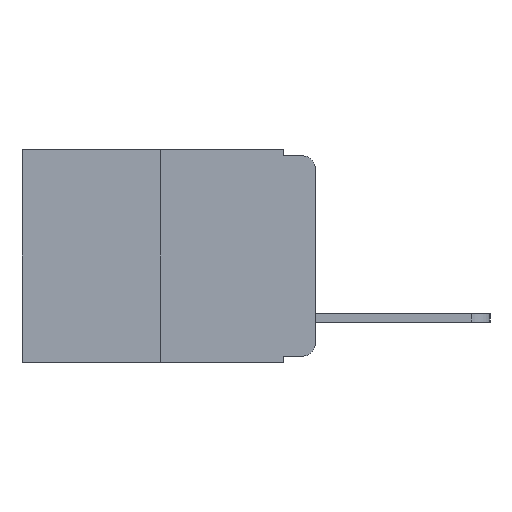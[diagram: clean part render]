
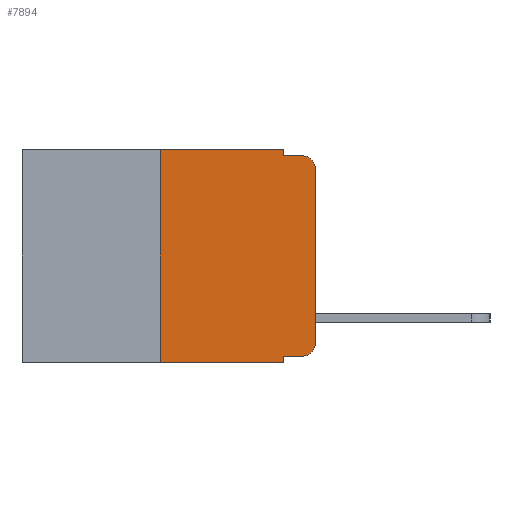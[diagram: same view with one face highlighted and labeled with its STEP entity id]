
A CAD part, left-side view. The second image highlights one B-rep face of the part: STEP entity #7894.
In plain terms, the highlighted planar face has unit normal (-1, 0, 0).
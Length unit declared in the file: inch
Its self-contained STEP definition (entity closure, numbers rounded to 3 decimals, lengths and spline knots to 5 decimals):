
#163 = AXIS2_PLACEMENT_3D ( 'NONE', #10218, #760, #6037 ) ;
#239 = EDGE_CURVE ( 'NONE', #9071, #713, #4498, .T. ) ;
#278 = VERTEX_POINT ( 'NONE', #9108 ) ;
#324 = VECTOR ( 'NONE', #2388, 39.37008 ) ;
#398 = DIRECTION ( 'NONE',  ( 0., 0., -1. ) ) ;
#529 = CARTESIAN_POINT ( 'NONE',  ( 0., 0.25, -0.343 ) ) ;
#713 = VERTEX_POINT ( 'NONE', #7970 ) ;
#725 = VERTEX_POINT ( 'NONE', #7679 ) ;
#760 = DIRECTION ( 'NONE',  ( 1., 0., 0. ) ) ;
#961 = EDGE_CURVE ( 'NONE', #4079, #9071, #7833, .T. ) ;
#1276 = FACE_OUTER_BOUND ( 'NONE', #2733, .T. ) ;
#1475 = LINE ( 'NONE', #11955, #6306 ) ;
#1564 = VERTEX_POINT ( 'NONE', #8216 ) ;
#1623 = PLANE ( 'NONE',  #163 ) ;
#2388 = DIRECTION ( 'NONE',  ( 0., 0., 1. ) ) ;
#2514 = LINE ( 'NONE', #10098, #7355 ) ;
#2542 = CARTESIAN_POINT ( 'NONE',  ( 0., 0., 0. ) ) ;
#2733 = EDGE_LOOP ( 'NONE', ( #9099, #9053, #7540, #7674, #8092, #8365, #9820, #9903, #7124, #10773 ) ) ;
#3201 = CARTESIAN_POINT ( 'NONE',  ( 0., 0.02, -0.333 ) ) ;
#3398 = VECTOR ( 'NONE', #6709, 39.37008 ) ;
#3698 = CARTESIAN_POINT ( 'NONE',  ( 0., 0.051, -0.01 ) ) ;
#4079 = VERTEX_POINT ( 'NONE', #12524 ) ;
#4468 = DIRECTION ( 'NONE',  ( 0., -1., 0. ) ) ;
#4474 = VERTEX_POINT ( 'NONE', #10710 ) ;
#4498 = CIRCLE ( 'NONE', #9310, 0.02 ) ;
#5006 = CARTESIAN_POINT ( 'NONE',  ( 0., 0.473, -0.343 ) ) ;
#5178 = VECTOR ( 'NONE', #5620, 39.37008 ) ;
#5368 = EDGE_CURVE ( 'NONE', #8167, #4474, #9248, .T. ) ;
#5620 = DIRECTION ( 'NONE',  ( 0., -1., 0. ) ) ;
#5674 = CARTESIAN_POINT ( 'NONE',  ( 0., 0.473, 0. ) ) ;
#5928 = CARTESIAN_POINT ( 'NONE',  ( 0., 0.051, 0. ) ) ;
#5963 = DIRECTION ( 'NONE',  ( 0., 0., -1. ) ) ;
#6037 = DIRECTION ( 'NONE',  ( 0., 0., -1. ) ) ;
#6229 = DIRECTION ( 'NONE',  ( 0., -1., 0. ) ) ;
#6306 = VECTOR ( 'NONE', #6229, 39.37008 ) ;
#6442 = EDGE_CURVE ( 'NONE', #7568, #4079, #12196, .T. ) ;
#6520 = CARTESIAN_POINT ( 'NONE',  ( 0., 0.02, -0.03 ) ) ;
#6709 = DIRECTION ( 'NONE',  ( 0., -1., 0. ) ) ;
#7108 = EDGE_CURVE ( 'NONE', #8213, #7568, #1475, .T. ) ;
#7124 = ORIENTED_EDGE ( 'NONE', *, *, #7108, .T. ) ;
#7355 = VECTOR ( 'NONE', #398, 39.37008 ) ;
#7428 = DIRECTION ( 'NONE',  ( 0., 0., -1. ) ) ;
#7532 = CARTESIAN_POINT ( 'NONE',  ( 0., 0.02, -0.313 ) ) ;
#7540 = ORIENTED_EDGE ( 'NONE', *, *, #11811, .F. ) ;
#7568 = VERTEX_POINT ( 'NONE', #3201 ) ;
#7674 = ORIENTED_EDGE ( 'NONE', *, *, #10619, .F. ) ;
#7679 = CARTESIAN_POINT ( 'NONE',  ( 0., 0.051, -0.01 ) ) ;
#7768 = LINE ( 'NONE', #3698, #5178 ) ;
#7822 = EDGE_CURVE ( 'NONE', #8213, #4474, #2514, .T. ) ;
#7833 = LINE ( 'NONE', #2542, #10894 ) ;
#7882 = DIRECTION ( 'NONE',  ( -1., 0., 0. ) ) ;
#7894 = ADVANCED_FACE ( 'NONE', ( #1276 ), #1623, .F. ) ;
#7936 = LINE ( 'NONE', #8284, #324 ) ;
#7970 = CARTESIAN_POINT ( 'NONE',  ( 0., 0.02, -0.01 ) ) ;
#8092 = ORIENTED_EDGE ( 'NONE', *, *, #8837, .F. ) ;
#8150 = AXIS2_PLACEMENT_3D ( 'NONE', #7532, #7882, #7428 ) ;
#8167 = VERTEX_POINT ( 'NONE', #529 ) ;
#8213 = VERTEX_POINT ( 'NONE', #12263 ) ;
#8216 = CARTESIAN_POINT ( 'NONE',  ( 0., 0.051, 0. ) ) ;
#8284 = CARTESIAN_POINT ( 'NONE',  ( 0., 0.25, 0. ) ) ;
#8294 = DIRECTION ( 'NONE',  ( 0., 0., -1. ) ) ;
#8365 = ORIENTED_EDGE ( 'NONE', *, *, #9949, .F. ) ;
#8547 = CARTESIAN_POINT ( 'NONE',  ( 0., 0., -0.03 ) ) ;
#8837 = EDGE_CURVE ( 'NONE', #278, #1564, #8968, .T. ) ;
#8968 = LINE ( 'NONE', #5674, #3398 ) ;
#9053 = ORIENTED_EDGE ( 'NONE', *, *, #239, .T. ) ;
#9071 = VERTEX_POINT ( 'NONE', #8547 ) ;
#9099 = ORIENTED_EDGE ( 'NONE', *, *, #961, .T. ) ;
#9108 = CARTESIAN_POINT ( 'NONE',  ( 0., 0.25, 0. ) ) ;
#9122 = LINE ( 'NONE', #5928, #11428 ) ;
#9248 = LINE ( 'NONE', #5006, #11523 ) ;
#9310 = AXIS2_PLACEMENT_3D ( 'NONE', #6520, #9426, #8294 ) ;
#9426 = DIRECTION ( 'NONE',  ( -1., 0., 0. ) ) ;
#9496 = DIRECTION ( 'NONE',  ( 0., 0., 1. ) ) ;
#9820 = ORIENTED_EDGE ( 'NONE', *, *, #5368, .T. ) ;
#9903 = ORIENTED_EDGE ( 'NONE', *, *, #7822, .F. ) ;
#9949 = EDGE_CURVE ( 'NONE', #8167, #278, #7936, .T. ) ;
#10098 = CARTESIAN_POINT ( 'NONE',  ( 0., 0.051, 0. ) ) ;
#10218 = CARTESIAN_POINT ( 'NONE',  ( 0., 0.473, 0. ) ) ;
#10619 = EDGE_CURVE ( 'NONE', #1564, #725, #9122, .T. ) ;
#10710 = CARTESIAN_POINT ( 'NONE',  ( 0., 0.051, -0.343 ) ) ;
#10773 = ORIENTED_EDGE ( 'NONE', *, *, #6442, .T. ) ;
#10894 = VECTOR ( 'NONE', #9496, 39.37008 ) ;
#11428 = VECTOR ( 'NONE', #5963, 39.37008 ) ;
#11523 = VECTOR ( 'NONE', #4468, 39.37008 ) ;
#11811 = EDGE_CURVE ( 'NONE', #725, #713, #7768, .T. ) ;
#11955 = CARTESIAN_POINT ( 'NONE',  ( 0., 0.051, -0.333 ) ) ;
#12196 = CIRCLE ( 'NONE', #8150, 0.02 ) ;
#12263 = CARTESIAN_POINT ( 'NONE',  ( 0., 0.051, -0.333 ) ) ;
#12524 = CARTESIAN_POINT ( 'NONE',  ( 0., 0., -0.313 ) ) ;
